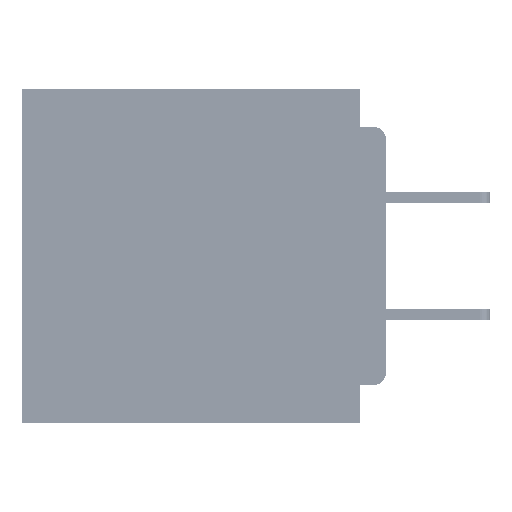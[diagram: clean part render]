
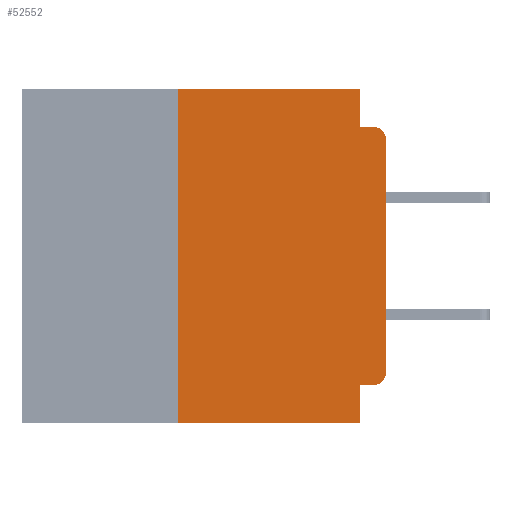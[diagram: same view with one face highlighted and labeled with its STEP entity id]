
A CAD part, left-side view. The second image highlights one B-rep face of the part: STEP entity #52552.
In plain terms, the highlighted planar face has unit normal (-1, 0, 0).
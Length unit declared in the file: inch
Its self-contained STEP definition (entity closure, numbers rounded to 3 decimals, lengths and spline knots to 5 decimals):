
#729 = CIRCLE ( 'NONE', #42034, 0.015 ) ;
#852 = CARTESIAN_POINT ( 'NONE',  ( 0., 0.031, 0. ) ) ;
#4084 = DIRECTION ( 'NONE',  ( 0., -1., 0. ) ) ;
#5014 = DIRECTION ( 'NONE',  ( 1., 0., 0. ) ) ;
#5420 = CARTESIAN_POINT ( 'NONE',  ( 0., 0., -0.045 ) ) ;
#6771 = CARTESIAN_POINT ( 'NONE',  ( 0., 0.031, -0.355 ) ) ;
#6954 = CARTESIAN_POINT ( 'NONE',  ( 0., 0.015, -0.34 ) ) ;
#7440 = VERTEX_POINT ( 'NONE', #10524 ) ;
#8008 = ORIENTED_EDGE ( 'NONE', *, *, #49681, .F. ) ;
#9532 = CARTESIAN_POINT ( 'NONE',  ( 0., 0.031, -0.045 ) ) ;
#10524 = CARTESIAN_POINT ( 'NONE',  ( 0., 0.25, 0. ) ) ;
#11465 = ORIENTED_EDGE ( 'NONE', *, *, #67672, .F. ) ;
#12367 = DIRECTION ( 'NONE',  ( 0., 0., -1. ) ) ;
#12524 = DIRECTION ( 'NONE',  ( 0., 0., -1. ) ) ;
#13475 = ORIENTED_EDGE ( 'NONE', *, *, #63299, .T. ) ;
#16240 = ORIENTED_EDGE ( 'NONE', *, *, #31166, .F. ) ;
#16642 = VECTOR ( 'NONE', #45572, 39.37008 ) ;
#17930 = CARTESIAN_POINT ( 'NONE',  ( 0., 0.031, -0.4 ) ) ;
#18030 = DIRECTION ( 'NONE',  ( 0., 0., 1. ) ) ;
#19114 = CARTESIAN_POINT ( 'NONE',  ( 0., 0.015, -0.355 ) ) ;
#19132 = VERTEX_POINT ( 'NONE', #62938 ) ;
#20916 = LINE ( 'NONE', #62163, #48499 ) ;
#21052 = CARTESIAN_POINT ( 'NONE',  ( 0., 0.25, -0.4 ) ) ;
#21550 = VECTOR ( 'NONE', #12367, 39.37008 ) ;
#23294 = LINE ( 'NONE', #17930, #21550 ) ;
#23295 = EDGE_CURVE ( 'NONE', #47436, #59983, #30085, .T. ) ;
#23597 = CARTESIAN_POINT ( 'NONE',  ( 0., 0.25, -0.4 ) ) ;
#23609 = CARTESIAN_POINT ( 'NONE',  ( 0., 0., 0. ) ) ;
#24142 = CARTESIAN_POINT ( 'NONE',  ( 0., 0., -0.355 ) ) ;
#26149 = ORIENTED_EDGE ( 'NONE', *, *, #32503, .T. ) ;
#26518 = VERTEX_POINT ( 'NONE', #852 ) ;
#27341 = DIRECTION ( 'NONE',  ( -1., 0., 0. ) ) ;
#28696 = VECTOR ( 'NONE', #44110, 39.37008 ) ;
#29519 = ORIENTED_EDGE ( 'NONE', *, *, #63021, .T. ) ;
#30085 = CIRCLE ( 'NONE', #68673, 0.015 ) ;
#31166 = EDGE_CURVE ( 'NONE', #60530, #59983, #43317, .T. ) ;
#31503 = CARTESIAN_POINT ( 'NONE',  ( 0., 0.437, -0.4 ) ) ;
#32226 = VERTEX_POINT ( 'NONE', #21052 ) ;
#32503 = EDGE_CURVE ( 'NONE', #45320, #44074, #729, .T. ) ;
#32924 = PLANE ( 'NONE',  #41778 ) ;
#34702 = EDGE_CURVE ( 'NONE', #45320, #56710, #50195, .T. ) ;
#34936 = LINE ( 'NONE', #23597, #62381 ) ;
#35565 = VECTOR ( 'NONE', #51814, 39.37008 ) ;
#35622 = CARTESIAN_POINT ( 'NONE',  ( 0., 0.015, -0.045 ) ) ;
#38691 = DIRECTION ( 'NONE',  ( 0., 0., -1. ) ) ;
#41778 = AXIS2_PLACEMENT_3D ( 'NONE', #49494, #5014, #38691 ) ;
#42034 = AXIS2_PLACEMENT_3D ( 'NONE', #6954, #45605, #12524 ) ;
#42729 = LINE ( 'NONE', #23609, #61557 ) ;
#43317 = LINE ( 'NONE', #5420, #28696 ) ;
#44074 = VERTEX_POINT ( 'NONE', #46530 ) ;
#44110 = DIRECTION ( 'NONE',  ( 0., -1., 0. ) ) ;
#45320 = VERTEX_POINT ( 'NONE', #19114 ) ;
#45572 = DIRECTION ( 'NONE',  ( 0., -1., 0. ) ) ;
#45605 = DIRECTION ( 'NONE',  ( -1., 0., 0. ) ) ;
#45962 = EDGE_LOOP ( 'NONE', ( #13475, #51463, #16240, #70624, #11465, #8008, #29519, #59148, #54570, #26149 ) ) ;
#46530 = CARTESIAN_POINT ( 'NONE',  ( 0., 0., -0.34 ) ) ;
#47436 = VERTEX_POINT ( 'NONE', #55454 ) ;
#48499 = VECTOR ( 'NONE', #67637, 39.37008 ) ;
#49494 = CARTESIAN_POINT ( 'NONE',  ( 0., 0.437, 0. ) ) ;
#49681 = EDGE_CURVE ( 'NONE', #32226, #7440, #34936, .T. ) ;
#50195 = LINE ( 'NONE', #24142, #35565 ) ;
#50828 = EDGE_CURVE ( 'NONE', #26518, #60530, #20916, .T. ) ;
#51463 = ORIENTED_EDGE ( 'NONE', *, *, #23295, .T. ) ;
#51814 = DIRECTION ( 'NONE',  ( 0., 1., 0. ) ) ;
#52175 = EDGE_CURVE ( 'NONE', #56710, #19132, #23294, .T. ) ;
#52552 = ADVANCED_FACE ( 'NONE', ( #59372 ), #32924, .F. ) ;
#54570 = ORIENTED_EDGE ( 'NONE', *, *, #34702, .F. ) ;
#55454 = CARTESIAN_POINT ( 'NONE',  ( 0., 0., -0.06 ) ) ;
#56443 = LINE ( 'NONE', #31503, #65887 ) ;
#56539 = DIRECTION ( 'NONE',  ( 0., 0., 1. ) ) ;
#56710 = VERTEX_POINT ( 'NONE', #6771 ) ;
#59148 = ORIENTED_EDGE ( 'NONE', *, *, #52175, .F. ) ;
#59372 = FACE_OUTER_BOUND ( 'NONE', #45962, .T. ) ;
#59983 = VERTEX_POINT ( 'NONE', #35622 ) ;
#60237 = CARTESIAN_POINT ( 'NONE',  ( 0., 0.015, -0.06 ) ) ;
#60530 = VERTEX_POINT ( 'NONE', #9532 ) ;
#60586 = LINE ( 'NONE', #67361, #16642 ) ;
#61557 = VECTOR ( 'NONE', #56539, 39.37008 ) ;
#62163 = CARTESIAN_POINT ( 'NONE',  ( 0., 0.031, 0. ) ) ;
#62381 = VECTOR ( 'NONE', #18030, 39.37008 ) ;
#62938 = CARTESIAN_POINT ( 'NONE',  ( 0., 0.031, -0.4 ) ) ;
#63021 = EDGE_CURVE ( 'NONE', #32226, #19132, #56443, .T. ) ;
#63299 = EDGE_CURVE ( 'NONE', #44074, #47436, #42729, .T. ) ;
#65755 = DIRECTION ( 'NONE',  ( 0., 0., -1. ) ) ;
#65887 = VECTOR ( 'NONE', #4084, 39.37008 ) ;
#67361 = CARTESIAN_POINT ( 'NONE',  ( 0., 0.437, 0. ) ) ;
#67637 = DIRECTION ( 'NONE',  ( 0., 0., -1. ) ) ;
#67672 = EDGE_CURVE ( 'NONE', #7440, #26518, #60586, .T. ) ;
#68673 = AXIS2_PLACEMENT_3D ( 'NONE', #60237, #27341, #65755 ) ;
#70624 = ORIENTED_EDGE ( 'NONE', *, *, #50828, .F. ) ;
